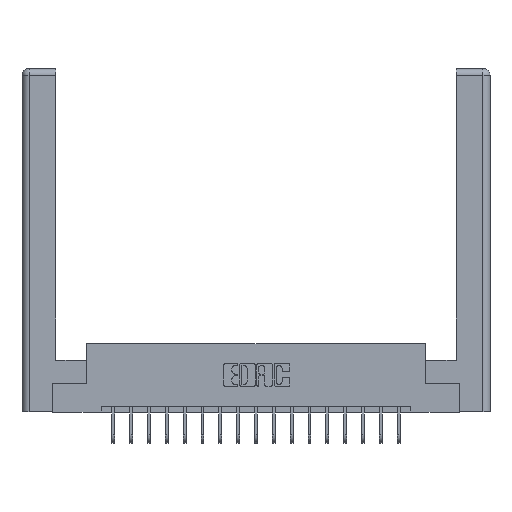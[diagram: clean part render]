
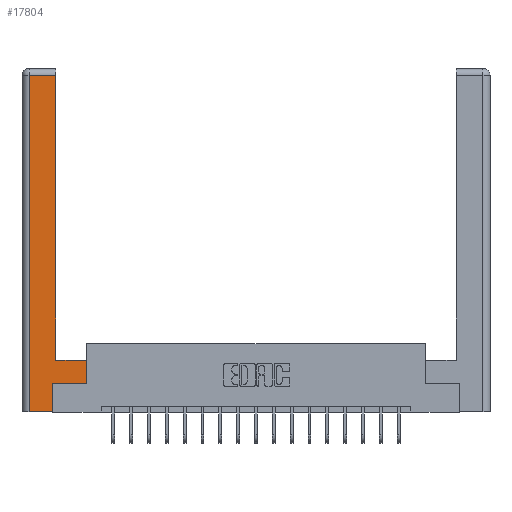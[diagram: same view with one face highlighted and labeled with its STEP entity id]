
A CAD part, top view. The second image highlights one B-rep face of the part: STEP entity #17804.
In plain terms, the highlighted planar face has unit normal (0, 0, 1).
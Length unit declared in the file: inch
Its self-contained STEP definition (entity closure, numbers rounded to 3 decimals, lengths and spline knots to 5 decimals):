
#522 = LINE ( 'NONE', #3920, #14488 ) ;
#847 = CARTESIAN_POINT ( 'NONE',  ( 0.0615, 2.94, 0. ) ) ;
#998 = ORIENTED_EDGE ( 'NONE', *, *, #11408, .T. ) ;
#1011 = VECTOR ( 'NONE', #6503, 39.37008 ) ;
#1262 = ORIENTED_EDGE ( 'NONE', *, *, #13006, .T. ) ;
#1364 = DIRECTION ( 'NONE',  ( -1., 0., 0. ) ) ;
#1705 = DIRECTION ( 'NONE',  ( 0., -1., 0. ) ) ;
#1906 = DIRECTION ( 'NONE',  ( 0., 1., 0. ) ) ;
#2052 = LINE ( 'NONE', #16944, #6169 ) ;
#3250 = CARTESIAN_POINT ( 'NONE',  ( 0.0615, 0., 0. ) ) ;
#3545 = EDGE_CURVE ( 'NONE', #12929, #8879, #10252, .T. ) ;
#3650 = VECTOR ( 'NONE', #11239, 39.37008 ) ;
#3884 = VECTOR ( 'NONE', #9626, 39.37008 ) ;
#3920 = CARTESIAN_POINT ( 'NONE',  ( 0.565, 0.245, 0. ) ) ;
#4138 = DIRECTION ( 'NONE',  ( 0., 0., -1. ) ) ;
#4780 = CARTESIAN_POINT ( 'NONE',  ( 0.295, 0.45, 0. ) ) ;
#5170 = VERTEX_POINT ( 'NONE', #13803 ) ;
#5698 = CARTESIAN_POINT ( 'NONE',  ( 0., 0., 0. ) ) ;
#6109 = ORIENTED_EDGE ( 'NONE', *, *, #15259, .T. ) ;
#6149 = CARTESIAN_POINT ( 'NONE',  ( 0.565, 0.45, 0. ) ) ;
#6169 = VECTOR ( 'NONE', #18490, 39.37008 ) ;
#6503 = DIRECTION ( 'NONE',  ( 0., 1., 0. ) ) ;
#6589 = EDGE_CURVE ( 'NONE', #12570, #5170, #15677, .T. ) ;
#6945 = CARTESIAN_POINT ( 'NONE',  ( 0.265, 0., 0. ) ) ;
#7073 = VECTOR ( 'NONE', #13814, 39.37008 ) ;
#7095 = EDGE_CURVE ( 'NONE', #11097, #8693, #17203, .T. ) ;
#7157 = EDGE_LOOP ( 'NONE', ( #6109, #10164, #18040, #1262, #15353, #998, #8104, #10896 ) ) ;
#7222 = LINE ( 'NONE', #6945, #3884 ) ;
#7340 = CARTESIAN_POINT ( 'NONE',  ( 0.565, 0.245, 0. ) ) ;
#7680 = CARTESIAN_POINT ( 'NONE',  ( 0.0615, 0., 0. ) ) ;
#7865 = FACE_OUTER_BOUND ( 'NONE', #7157, .T. ) ;
#8104 = ORIENTED_EDGE ( 'NONE', *, *, #7095, .T. ) ;
#8272 = VECTOR ( 'NONE', #1906, 39.37008 ) ;
#8693 = VERTEX_POINT ( 'NONE', #6149 ) ;
#8879 = VERTEX_POINT ( 'NONE', #7680 ) ;
#9075 = CARTESIAN_POINT ( 'NONE',  ( 0.265, 0., 0. ) ) ;
#9579 = LINE ( 'NONE', #10938, #7073 ) ;
#9626 = DIRECTION ( 'NONE',  ( 1., 0., 0. ) ) ;
#9719 = DIRECTION ( 'NONE',  ( 1., 0., 0. ) ) ;
#9723 = AXIS2_PLACEMENT_3D ( 'NONE', #5698, #4138, #1364 ) ;
#10164 = ORIENTED_EDGE ( 'NONE', *, *, #15970, .T. ) ;
#10165 = EDGE_CURVE ( 'NONE', #8693, #13288, #11347, .T. ) ;
#10252 = LINE ( 'NONE', #3250, #12498 ) ;
#10896 = ORIENTED_EDGE ( 'NONE', *, *, #10165, .T. ) ;
#10938 = CARTESIAN_POINT ( 'NONE',  ( 0.295, 3., 0. ) ) ;
#11097 = VERTEX_POINT ( 'NONE', #7340 ) ;
#11239 = DIRECTION ( 'NONE',  ( -1., 0., 0. ) ) ;
#11347 = LINE ( 'NONE', #12587, #3650 ) ;
#11408 = EDGE_CURVE ( 'NONE', #5170, #11097, #522, .T. ) ;
#12498 = VECTOR ( 'NONE', #1705, 39.37008 ) ;
#12570 = VERTEX_POINT ( 'NONE', #9075 ) ;
#12587 = CARTESIAN_POINT ( 'NONE',  ( 0.295, 0.45, 0. ) ) ;
#12929 = VERTEX_POINT ( 'NONE', #847 ) ;
#13006 = EDGE_CURVE ( 'NONE', #8879, #12570, #7222, .T. ) ;
#13288 = VERTEX_POINT ( 'NONE', #4780 ) ;
#13803 = CARTESIAN_POINT ( 'NONE',  ( 0.265, 0.245, 0. ) ) ;
#13814 = DIRECTION ( 'NONE',  ( 0., 1., 0. ) ) ;
#13816 = CARTESIAN_POINT ( 'NONE',  ( 0.565, 0.45, 0. ) ) ;
#14488 = VECTOR ( 'NONE', #9719, 39.37008 ) ;
#15259 = EDGE_CURVE ( 'NONE', #13288, #18499, #9579, .T. ) ;
#15353 = ORIENTED_EDGE ( 'NONE', *, *, #6589, .T. ) ;
#15677 = LINE ( 'NONE', #15932, #8272 ) ;
#15932 = CARTESIAN_POINT ( 'NONE',  ( 0.265, 0.245, 0. ) ) ;
#15970 = EDGE_CURVE ( 'NONE', #18499, #12929, #2052, .T. ) ;
#16944 = CARTESIAN_POINT ( 'NONE',  ( 0.0615, 2.94, 0. ) ) ;
#17203 = LINE ( 'NONE', #13816, #1011 ) ;
#17804 = ADVANCED_FACE ( 'NONE', ( #7865 ), #18396, .F. ) ;
#18040 = ORIENTED_EDGE ( 'NONE', *, *, #3545, .T. ) ;
#18396 = PLANE ( 'NONE',  #9723 ) ;
#18490 = DIRECTION ( 'NONE',  ( -1., 0., 0. ) ) ;
#18499 = VERTEX_POINT ( 'NONE', #18555 ) ;
#18555 = CARTESIAN_POINT ( 'NONE',  ( 0.295, 2.94, 0. ) ) ;
